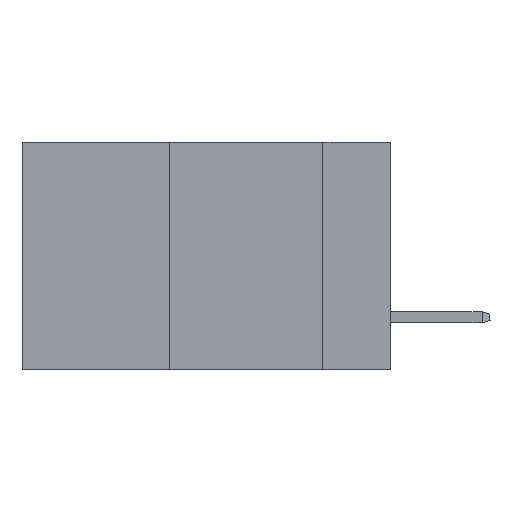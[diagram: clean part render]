
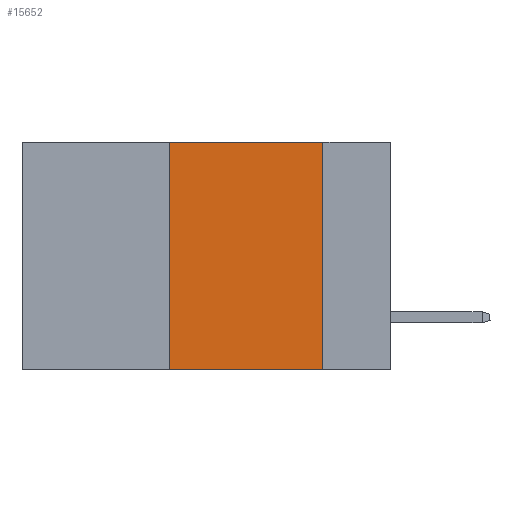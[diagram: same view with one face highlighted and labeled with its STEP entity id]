
A CAD part, left-side view. The second image highlights one B-rep face of the part: STEP entity #15652.
In plain terms, the highlighted planar face has unit normal (-1, 0, 0).
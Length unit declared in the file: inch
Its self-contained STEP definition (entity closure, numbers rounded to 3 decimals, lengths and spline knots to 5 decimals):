
#64 = VECTOR ( 'NONE', #1520, 39.37008 ) ;
#178 = VERTEX_POINT ( 'NONE', #11643 ) ;
#951 = CARTESIAN_POINT ( 'NONE',  ( 0., 0.6, 0. ) ) ;
#1019 = DIRECTION ( 'NONE',  ( 0., -1., 0. ) ) ;
#1117 = EDGE_CURVE ( 'NONE', #178, #12737, #15674, .T. ) ;
#1214 = CARTESIAN_POINT ( 'NONE',  ( 0., 0.36, 0. ) ) ;
#1386 = CARTESIAN_POINT ( 'NONE',  ( 0., 0.6, 0. ) ) ;
#1505 = PLANE ( 'NONE',  #10116 ) ;
#1520 = DIRECTION ( 'NONE',  ( 0., 0., -1. ) ) ;
#2858 = CARTESIAN_POINT ( 'NONE',  ( 0., 0.36, 0. ) ) ;
#3666 = DIRECTION ( 'NONE',  ( 0., 0., 1. ) ) ;
#4316 = VECTOR ( 'NONE', #3666, 39.37008 ) ;
#4911 = EDGE_CURVE ( 'NONE', #11342, #12737, #13163, .T. ) ;
#5724 = CARTESIAN_POINT ( 'NONE',  ( 0., 0.6, -0.37 ) ) ;
#6202 = CARTESIAN_POINT ( 'NONE',  ( 0., 0.36, -0.37 ) ) ;
#6654 = EDGE_LOOP ( 'NONE', ( #9534, #9032, #12229, #14508 ) ) ;
#6919 = DIRECTION ( 'NONE',  ( 1., 0., 0. ) ) ;
#7677 = VECTOR ( 'NONE', #1019, 39.37008 ) ;
#8689 = VECTOR ( 'NONE', #14781, 39.37008 ) ;
#8769 = CARTESIAN_POINT ( 'NONE',  ( 0., 0.11, 0. ) ) ;
#9032 = ORIENTED_EDGE ( 'NONE', *, *, #9470, .F. ) ;
#9470 = EDGE_CURVE ( 'NONE', #9947, #178, #11870, .T. ) ;
#9534 = ORIENTED_EDGE ( 'NONE', *, *, #1117, .F. ) ;
#9947 = VERTEX_POINT ( 'NONE', #2858 ) ;
#10116 = AXIS2_PLACEMENT_3D ( 'NONE', #951, #6919, #12212 ) ;
#11133 = LINE ( 'NONE', #1214, #4316 ) ;
#11342 = VERTEX_POINT ( 'NONE', #6202 ) ;
#11643 = CARTESIAN_POINT ( 'NONE',  ( 0., 0.11, 0. ) ) ;
#11870 = LINE ( 'NONE', #1386, #8689 ) ;
#12211 = FACE_OUTER_BOUND ( 'NONE', #6654, .T. ) ;
#12212 = DIRECTION ( 'NONE',  ( 0., 0., -1. ) ) ;
#12229 = ORIENTED_EDGE ( 'NONE', *, *, #14556, .F. ) ;
#12737 = VERTEX_POINT ( 'NONE', #12827 ) ;
#12827 = CARTESIAN_POINT ( 'NONE',  ( 0., 0.11, -0.37 ) ) ;
#13163 = LINE ( 'NONE', #5724, #7677 ) ;
#14508 = ORIENTED_EDGE ( 'NONE', *, *, #4911, .T. ) ;
#14556 = EDGE_CURVE ( 'NONE', #11342, #9947, #11133, .T. ) ;
#14781 = DIRECTION ( 'NONE',  ( 0., -1., 0. ) ) ;
#15652 = ADVANCED_FACE ( 'NONE', ( #12211 ), #1505, .F. ) ;
#15674 = LINE ( 'NONE', #8769, #64 ) ;
